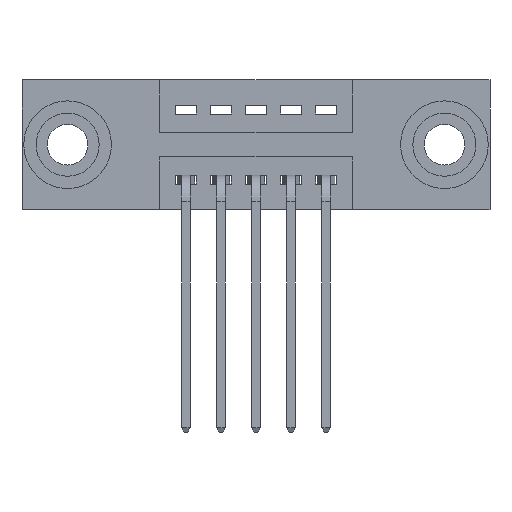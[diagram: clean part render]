
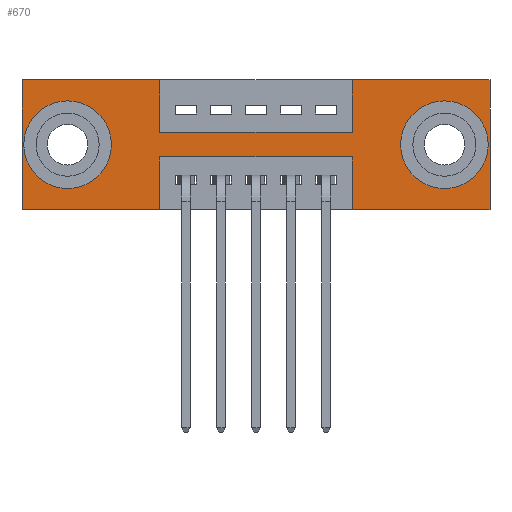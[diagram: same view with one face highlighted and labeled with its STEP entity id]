
A CAD part, front view. The second image highlights one B-rep face of the part: STEP entity #670.
In plain terms, the highlighted planar face has unit normal (0, -1, 0).
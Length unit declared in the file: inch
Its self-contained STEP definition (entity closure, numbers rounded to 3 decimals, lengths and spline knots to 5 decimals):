
#1 = VECTOR ( 'NONE', #2769, 39.37008 ) ;
#23 = VECTOR ( 'NONE', #7403, 39.37008 ) ;
#102 = DIRECTION ( 'NONE',  ( 1., 0., 0. ) ) ;
#108 = VECTOR ( 'NONE', #5703, 39.37008 ) ;
#118 = CARTESIAN_POINT ( 'NONE',  ( 1.335, 0., 0. ) ) ;
#206 = DIRECTION ( 'NONE',  ( 0., 0., -1. ) ) ;
#352 = DIRECTION ( 'NONE',  ( 1., 0., 0. ) ) ;
#407 = AXIS2_PLACEMENT_3D ( 'NONE', #7562, #2498, #3916 ) ;
#428 = ORIENTED_EDGE ( 'NONE', *, *, #5043, .F. ) ;
#445 = CIRCLE ( 'NONE', #8987, 0.078 ) ;
#455 = CARTESIAN_POINT ( 'NONE',  ( 0., 0., 0. ) ) ;
#481 = DIRECTION ( 'NONE',  ( 1., 0., 0. ) ) ;
#486 = CARTESIAN_POINT ( 'NONE',  ( 0.9425, 0., -0.22 ) ) ;
#495 = CARTESIAN_POINT ( 'NONE',  ( 0.13, 0., -0.107 ) ) ;
#578 = EDGE_CURVE ( 'NONE', #4786, #4952, #3858, .T. ) ;
#613 = EDGE_CURVE ( 'NONE', #4952, #846, #3188, .T. ) ;
#647 = CARTESIAN_POINT ( 'NONE',  ( 0., 0., -0.37 ) ) ;
#670 = ADVANCED_FACE ( 'NONE', ( #8381, #3408, #5368 ), #1763, .T. ) ;
#780 = LINE ( 'NONE', #9090, #8011 ) ;
#846 = VERTEX_POINT ( 'NONE', #7885 ) ;
#873 = ORIENTED_EDGE ( 'NONE', *, *, #5930, .T. ) ;
#910 = DIRECTION ( 'NONE',  ( 0., 1., 0. ) ) ;
#992 = EDGE_CURVE ( 'NONE', #7709, #9379, #3614, .T. ) ;
#993 = ORIENTED_EDGE ( 'NONE', *, *, #8884, .T. ) ;
#1116 = VERTEX_POINT ( 'NONE', #4364 ) ;
#1130 = CARTESIAN_POINT ( 'NONE',  ( 0.9425, 0., -0.15 ) ) ;
#1179 = CARTESIAN_POINT ( 'NONE',  ( 1.335, 0., -0.37 ) ) ;
#1230 = VERTEX_POINT ( 'NONE', #3477 ) ;
#1251 = VECTOR ( 'NONE', #2439, 39.37008 ) ;
#1307 = LINE ( 'NONE', #6205, #8888 ) ;
#1319 = CARTESIAN_POINT ( 'NONE',  ( 0.3925, 0., -0.15 ) ) ;
#1396 = CARTESIAN_POINT ( 'NONE',  ( 0.9425, 0., -0.37 ) ) ;
#1525 = DIRECTION ( 'NONE',  ( 0., 1., 0. ) ) ;
#1537 = EDGE_CURVE ( 'NONE', #3087, #9292, #8921, .T. ) ;
#1630 = CARTESIAN_POINT ( 'NONE',  ( 1.205, 0., -0.263 ) ) ;
#1677 = VERTEX_POINT ( 'NONE', #7965 ) ;
#1717 = LINE ( 'NONE', #455, #5623 ) ;
#1763 = PLANE ( 'NONE',  #6527 ) ;
#1818 = EDGE_LOOP ( 'NONE', ( #7102, #993 ) ) ;
#1851 = ORIENTED_EDGE ( 'NONE', *, *, #8972, .F. ) ;
#1888 = EDGE_CURVE ( 'NONE', #4394, #1116, #780, .T. ) ;
#1929 = DIRECTION ( 'NONE',  ( -1., 0., 0. ) ) ;
#1965 = CARTESIAN_POINT ( 'NONE',  ( 0.3925, 0., -0.22 ) ) ;
#2024 = DIRECTION ( 'NONE',  ( 0., 1., 0. ) ) ;
#2063 = VECTOR ( 'NONE', #102, 39.37008 ) ;
#2259 = VECTOR ( 'NONE', #206, 39.37008 ) ;
#2279 = CARTESIAN_POINT ( 'NONE',  ( 0.13, 0., -0.185 ) ) ;
#2439 = DIRECTION ( 'NONE',  ( -1., 0., 0. ) ) ;
#2498 = DIRECTION ( 'NONE',  ( 0., 1., 0. ) ) ;
#2554 = VERTEX_POINT ( 'NONE', #8993 ) ;
#2569 = DIRECTION ( 'NONE',  ( 0., -1., 0. ) ) ;
#2652 = LINE ( 'NONE', #6053, #2063 ) ;
#2695 = CARTESIAN_POINT ( 'NONE',  ( 0., 0., 0. ) ) ;
#2743 = AXIS2_PLACEMENT_3D ( 'NONE', #2773, #2024, #4976 ) ;
#2748 = VERTEX_POINT ( 'NONE', #1130 ) ;
#2769 = DIRECTION ( 'NONE',  ( 0., 0., 1. ) ) ;
#2773 = CARTESIAN_POINT ( 'NONE',  ( 0.13, 0., -0.185 ) ) ;
#3087 = VERTEX_POINT ( 'NONE', #495 ) ;
#3188 = LINE ( 'NONE', #5999, #1251 ) ;
#3408 = FACE_BOUND ( 'NONE', #8714, .T. ) ;
#3477 = CARTESIAN_POINT ( 'NONE',  ( 0.9425, 0., 0. ) ) ;
#3531 = CARTESIAN_POINT ( 'NONE',  ( 0., 0., 0. ) ) ;
#3579 = EDGE_LOOP ( 'NONE', ( #6616, #4598, #428, #3809, #4895, #8648, #3922, #3867, #8986, #8167, #1851, #6851 ) ) ;
#3614 = LINE ( 'NONE', #8006, #108 ) ;
#3651 = EDGE_CURVE ( 'NONE', #1230, #4786, #6706, .T. ) ;
#3713 = CARTESIAN_POINT ( 'NONE',  ( 0.13, 0., -0.263 ) ) ;
#3740 = VERTEX_POINT ( 'NONE', #1630 ) ;
#3773 = CIRCLE ( 'NONE', #4738, 0.078 ) ;
#3788 = LINE ( 'NONE', #7245, #7635 ) ;
#3809 = ORIENTED_EDGE ( 'NONE', *, *, #613, .F. ) ;
#3858 = LINE ( 'NONE', #118, #2259 ) ;
#3867 = ORIENTED_EDGE ( 'NONE', *, *, #4653, .F. ) ;
#3916 = DIRECTION ( 'NONE',  ( 0., 0., -1. ) ) ;
#3922 = ORIENTED_EDGE ( 'NONE', *, *, #4458, .F. ) ;
#4019 = CARTESIAN_POINT ( 'NONE',  ( 0., 0., -0.37 ) ) ;
#4043 = EDGE_CURVE ( 'NONE', #9379, #2554, #3788, .T. ) ;
#4364 = CARTESIAN_POINT ( 'NONE',  ( 0.3925, 0., 0. ) ) ;
#4387 = VERTEX_POINT ( 'NONE', #647 ) ;
#4394 = VERTEX_POINT ( 'NONE', #3531 ) ;
#4458 = EDGE_CURVE ( 'NONE', #2748, #1230, #6206, .T. ) ;
#4552 = DIRECTION ( 'NONE',  ( 0., 0., 1. ) ) ;
#4571 = LINE ( 'NONE', #1396, #1 ) ;
#4598 = ORIENTED_EDGE ( 'NONE', *, *, #992, .F. ) ;
#4653 = EDGE_CURVE ( 'NONE', #5739, #2748, #2652, .T. ) ;
#4738 = AXIS2_PLACEMENT_3D ( 'NONE', #7415, #1525, #6014 ) ;
#4786 = VERTEX_POINT ( 'NONE', #8356 ) ;
#4895 = ORIENTED_EDGE ( 'NONE', *, *, #578, .F. ) ;
#4952 = VERTEX_POINT ( 'NONE', #1179 ) ;
#4976 = DIRECTION ( 'NONE',  ( 0., 0., 1. ) ) ;
#5043 = EDGE_CURVE ( 'NONE', #846, #7709, #4571, .T. ) ;
#5105 = DIRECTION ( 'NONE',  ( 0., 0., -1. ) ) ;
#5203 = CARTESIAN_POINT ( 'NONE',  ( 0.3925, 0., 0. ) ) ;
#5263 = EDGE_CURVE ( 'NONE', #1116, #5739, #5816, .T. ) ;
#5368 = FACE_OUTER_BOUND ( 'NONE', #3579, .T. ) ;
#5550 = DIRECTION ( 'NONE',  ( 0., 0., 1. ) ) ;
#5623 = VECTOR ( 'NONE', #5550, 39.37008 ) ;
#5703 = DIRECTION ( 'NONE',  ( -1., 0., 0. ) ) ;
#5739 = VERTEX_POINT ( 'NONE', #1319 ) ;
#5816 = LINE ( 'NONE', #5203, #6109 ) ;
#5930 = EDGE_CURVE ( 'NONE', #9292, #3087, #445, .T. ) ;
#5999 = CARTESIAN_POINT ( 'NONE',  ( 0., 0., -0.37 ) ) ;
#6014 = DIRECTION ( 'NONE',  ( 0., 0., -1. ) ) ;
#6053 = CARTESIAN_POINT ( 'NONE',  ( 0.3925, 0., -0.15 ) ) ;
#6109 = VECTOR ( 'NONE', #5105, 39.37008 ) ;
#6205 = CARTESIAN_POINT ( 'NONE',  ( 0., 0., -0.37 ) ) ;
#6206 = LINE ( 'NONE', #8867, #23 ) ;
#6462 = DIRECTION ( 'NONE',  ( 0., 0., -1. ) ) ;
#6507 = ORIENTED_EDGE ( 'NONE', *, *, #1537, .T. ) ;
#6527 = AXIS2_PLACEMENT_3D ( 'NONE', #4019, #2569, #7727 ) ;
#6616 = ORIENTED_EDGE ( 'NONE', *, *, #4043, .F. ) ;
#6706 = LINE ( 'NONE', #2695, #6818 ) ;
#6818 = VECTOR ( 'NONE', #481, 39.37008 ) ;
#6851 = ORIENTED_EDGE ( 'NONE', *, *, #7525, .F. ) ;
#7102 = ORIENTED_EDGE ( 'NONE', *, *, #7496, .T. ) ;
#7245 = CARTESIAN_POINT ( 'NONE',  ( 0.3925, 0., -0.37 ) ) ;
#7403 = DIRECTION ( 'NONE',  ( 0., 0., 1. ) ) ;
#7415 = CARTESIAN_POINT ( 'NONE',  ( 1.205, 0., -0.185 ) ) ;
#7496 = EDGE_CURVE ( 'NONE', #1677, #3740, #8098, .T. ) ;
#7525 = EDGE_CURVE ( 'NONE', #2554, #4387, #1307, .T. ) ;
#7562 = CARTESIAN_POINT ( 'NONE',  ( 1.205, 0., -0.185 ) ) ;
#7635 = VECTOR ( 'NONE', #6462, 39.37008 ) ;
#7709 = VERTEX_POINT ( 'NONE', #486 ) ;
#7727 = DIRECTION ( 'NONE',  ( 0., 0., -1. ) ) ;
#7885 = CARTESIAN_POINT ( 'NONE',  ( 0.9425, 0., -0.37 ) ) ;
#7965 = CARTESIAN_POINT ( 'NONE',  ( 1.205, 0., -0.107 ) ) ;
#8006 = CARTESIAN_POINT ( 'NONE',  ( 0.3925, 0., -0.22 ) ) ;
#8011 = VECTOR ( 'NONE', #352, 39.37008 ) ;
#8098 = CIRCLE ( 'NONE', #407, 0.078 ) ;
#8167 = ORIENTED_EDGE ( 'NONE', *, *, #1888, .F. ) ;
#8356 = CARTESIAN_POINT ( 'NONE',  ( 1.335, 0., 0. ) ) ;
#8381 = FACE_BOUND ( 'NONE', #1818, .T. ) ;
#8648 = ORIENTED_EDGE ( 'NONE', *, *, #3651, .F. ) ;
#8714 = EDGE_LOOP ( 'NONE', ( #6507, #873 ) ) ;
#8867 = CARTESIAN_POINT ( 'NONE',  ( 0.9425, 0., 0. ) ) ;
#8884 = EDGE_CURVE ( 'NONE', #3740, #1677, #3773, .T. ) ;
#8888 = VECTOR ( 'NONE', #1929, 39.37008 ) ;
#8921 = CIRCLE ( 'NONE', #2743, 0.078 ) ;
#8972 = EDGE_CURVE ( 'NONE', #4387, #4394, #1717, .T. ) ;
#8986 = ORIENTED_EDGE ( 'NONE', *, *, #5263, .F. ) ;
#8987 = AXIS2_PLACEMENT_3D ( 'NONE', #2279, #910, #4552 ) ;
#8993 = CARTESIAN_POINT ( 'NONE',  ( 0.3925, 0., -0.37 ) ) ;
#9090 = CARTESIAN_POINT ( 'NONE',  ( 0., 0., 0. ) ) ;
#9292 = VERTEX_POINT ( 'NONE', #3713 ) ;
#9379 = VERTEX_POINT ( 'NONE', #1965 ) ;
